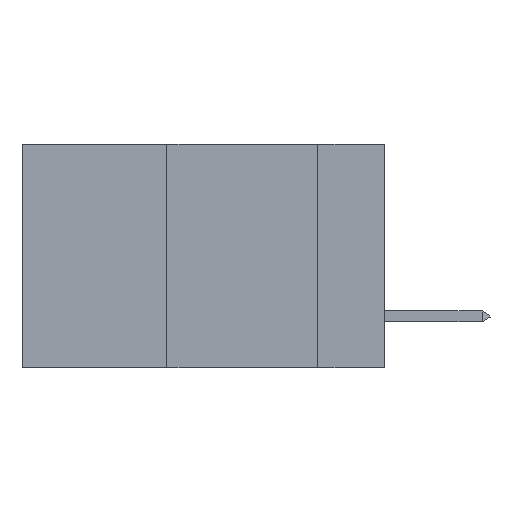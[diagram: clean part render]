
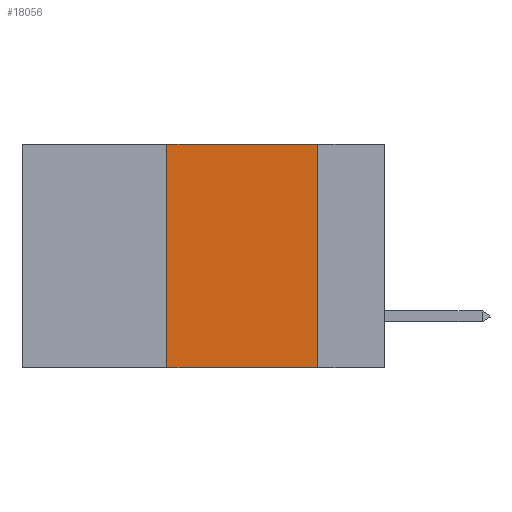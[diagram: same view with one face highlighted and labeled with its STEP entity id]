
A CAD part, left-side view. The second image highlights one B-rep face of the part: STEP entity #18056.
In plain terms, the highlighted planar face has unit normal (-1, 0, 0).
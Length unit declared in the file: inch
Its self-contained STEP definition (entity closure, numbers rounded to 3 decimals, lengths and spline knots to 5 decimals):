
#406 = FACE_OUTER_BOUND ( 'NONE', #11497, .T. ) ;
#1407 = DIRECTION ( 'NONE',  ( 0., -1., 0. ) ) ;
#2074 = LINE ( 'NONE', #25930, #20998 ) ;
#2327 = VERTEX_POINT ( 'NONE', #44339 ) ;
#3829 = ORIENTED_EDGE ( 'NONE', *, *, #20020, .F. ) ;
#4393 = LINE ( 'NONE', #41163, #9156 ) ;
#7115 = ORIENTED_EDGE ( 'NONE', *, *, #38940, .F. ) ;
#9156 = VECTOR ( 'NONE', #13758, 39.37008 ) ;
#9273 = CARTESIAN_POINT ( 'NONE',  ( 0., 0.11, 0. ) ) ;
#10221 = CARTESIAN_POINT ( 'NONE',  ( 0., 0.36, 0. ) ) ;
#11497 = EDGE_LOOP ( 'NONE', ( #20297, #3829, #7115, #40423 ) ) ;
#12723 = EDGE_CURVE ( 'NONE', #47294, #34771, #46251, .T. ) ;
#12986 = VECTOR ( 'NONE', #1407, 39.37008 ) ;
#13073 = DIRECTION ( 'NONE',  ( 0., 0., -1. ) ) ;
#13521 = PLANE ( 'NONE',  #35838 ) ;
#13758 = DIRECTION ( 'NONE',  ( 0., -1., 0. ) ) ;
#14845 = LINE ( 'NONE', #20428, #12986 ) ;
#15754 = CARTESIAN_POINT ( 'NONE',  ( 0., 0.11, -0.37 ) ) ;
#18056 = ADVANCED_FACE ( 'NONE', ( #406 ), #13521, .F. ) ;
#20020 = EDGE_CURVE ( 'NONE', #34681, #47294, #4393, .T. ) ;
#20297 = ORIENTED_EDGE ( 'NONE', *, *, #12723, .F. ) ;
#20428 = CARTESIAN_POINT ( 'NONE',  ( 0., 0.6, -0.37 ) ) ;
#20998 = VECTOR ( 'NONE', #48802, 39.37008 ) ;
#21334 = VECTOR ( 'NONE', #13073, 39.37008 ) ;
#22341 = EDGE_CURVE ( 'NONE', #2327, #34771, #14845, .T. ) ;
#24420 = CARTESIAN_POINT ( 'NONE',  ( 0., 0.6, 0. ) ) ;
#25930 = CARTESIAN_POINT ( 'NONE',  ( 0., 0.36, 0. ) ) ;
#26798 = CARTESIAN_POINT ( 'NONE',  ( 0., 0.11, 0. ) ) ;
#32416 = DIRECTION ( 'NONE',  ( 0., 0., -1. ) ) ;
#34681 = VERTEX_POINT ( 'NONE', #10221 ) ;
#34771 = VERTEX_POINT ( 'NONE', #15754 ) ;
#35838 = AXIS2_PLACEMENT_3D ( 'NONE', #24420, #43536, #32416 ) ;
#38940 = EDGE_CURVE ( 'NONE', #2327, #34681, #2074, .T. ) ;
#40423 = ORIENTED_EDGE ( 'NONE', *, *, #22341, .T. ) ;
#41163 = CARTESIAN_POINT ( 'NONE',  ( 0., 0.6, 0. ) ) ;
#43536 = DIRECTION ( 'NONE',  ( 1., 0., 0. ) ) ;
#44339 = CARTESIAN_POINT ( 'NONE',  ( 0., 0.36, -0.37 ) ) ;
#46251 = LINE ( 'NONE', #9273, #21334 ) ;
#47294 = VERTEX_POINT ( 'NONE', #26798 ) ;
#48802 = DIRECTION ( 'NONE',  ( 0., 0., 1. ) ) ;
